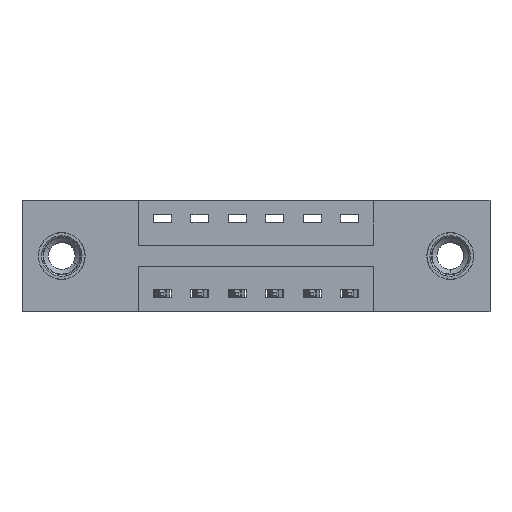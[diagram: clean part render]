
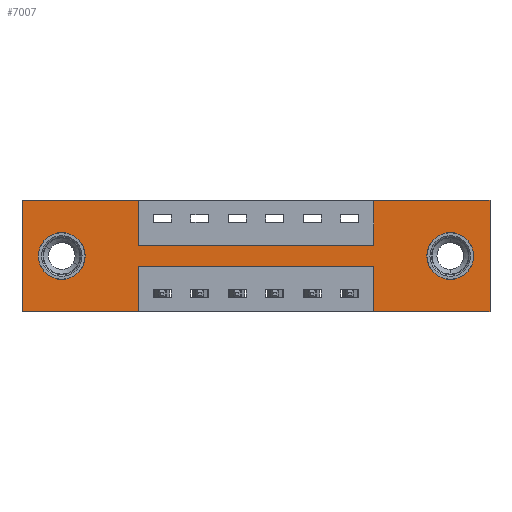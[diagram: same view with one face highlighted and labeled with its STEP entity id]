
A CAD part, front view. The second image highlights one B-rep face of the part: STEP entity #7007.
In plain terms, the highlighted planar face has unit normal (0, -1, 0).
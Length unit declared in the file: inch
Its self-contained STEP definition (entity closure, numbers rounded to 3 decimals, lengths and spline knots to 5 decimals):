
#60 = PLANE ( 'NONE',  #9162 ) ;
#218 = VERTEX_POINT ( 'NONE', #9192 ) ;
#221 = DIRECTION ( 'NONE',  ( 0., 0., 1. ) ) ;
#252 = AXIS2_PLACEMENT_3D ( 'NONE', #3395, #7339, #2103 ) ;
#494 = CARTESIAN_POINT ( 'NONE',  ( 1.56, 0., -0.37 ) ) ;
#575 = EDGE_CURVE ( 'NONE', #1447, #1108, #4317, .T. ) ;
#617 = DIRECTION ( 'NONE',  ( 0., 0., -1. ) ) ;
#659 = CARTESIAN_POINT ( 'NONE',  ( 0., 0., -0.37 ) ) ;
#671 = ORIENTED_EDGE ( 'NONE', *, *, #3765, .F. ) ;
#778 = ORIENTED_EDGE ( 'NONE', *, *, #8247, .F. ) ;
#977 = LINE ( 'NONE', #2435, #4681 ) ;
#992 = LINE ( 'NONE', #3208, #8016 ) ;
#1108 = VERTEX_POINT ( 'NONE', #1292 ) ;
#1255 = ORIENTED_EDGE ( 'NONE', *, *, #1481, .F. ) ;
#1270 = VECTOR ( 'NONE', #5062, 39.37008 ) ;
#1292 = CARTESIAN_POINT ( 'NONE',  ( 0.3875, 0., -0.37 ) ) ;
#1352 = VERTEX_POINT ( 'NONE', #8422 ) ;
#1397 = DIRECTION ( 'NONE',  ( -1., 0., 0. ) ) ;
#1408 = CARTESIAN_POINT ( 'NONE',  ( 1.4275, 0., -0.185 ) ) ;
#1447 = VERTEX_POINT ( 'NONE', #5711 ) ;
#1481 = EDGE_CURVE ( 'NONE', #1352, #1447, #5524, .T. ) ;
#1597 = CARTESIAN_POINT ( 'NONE',  ( 0.1325, 0., -0.107 ) ) ;
#1682 = CARTESIAN_POINT ( 'NONE',  ( 1.56, 0., 0. ) ) ;
#1745 = CIRCLE ( 'NONE', #7220, 0.078 ) ;
#1854 = CARTESIAN_POINT ( 'NONE',  ( 1.1725, 0., -0.37 ) ) ;
#1935 = CARTESIAN_POINT ( 'NONE',  ( 0.3875, 0., -0.15 ) ) ;
#1977 = DIRECTION ( 'NONE',  ( 0., 0., -1. ) ) ;
#2103 = DIRECTION ( 'NONE',  ( 0., 0., 1. ) ) ;
#2219 = VECTOR ( 'NONE', #9216, 39.37008 ) ;
#2435 = CARTESIAN_POINT ( 'NONE',  ( 1.1725, 0., 0. ) ) ;
#2485 = LINE ( 'NONE', #7800, #6066 ) ;
#2497 = DIRECTION ( 'NONE',  ( 0., 0., -1. ) ) ;
#2547 = VERTEX_POINT ( 'NONE', #1935 ) ;
#2572 = CARTESIAN_POINT ( 'NONE',  ( 0., 0., 0. ) ) ;
#2599 = ORIENTED_EDGE ( 'NONE', *, *, #575, .F. ) ;
#2664 = CARTESIAN_POINT ( 'NONE',  ( 0.1325, 0., -0.185 ) ) ;
#2705 = VECTOR ( 'NONE', #4104, 39.37008 ) ;
#2796 = VERTEX_POINT ( 'NONE', #7964 ) ;
#2830 = CIRCLE ( 'NONE', #8495, 0.078 ) ;
#2848 = AXIS2_PLACEMENT_3D ( 'NONE', #2664, #2879, #8687 ) ;
#2854 = CIRCLE ( 'NONE', #2848, 0.078 ) ;
#2879 = DIRECTION ( 'NONE',  ( 0., 1., 0. ) ) ;
#2963 = DIRECTION ( 'NONE',  ( 1., 0., 0. ) ) ;
#3015 = DIRECTION ( 'NONE',  ( 0., 0., -1. ) ) ;
#3023 = FACE_BOUND ( 'NONE', #6257, .T. ) ;
#3056 = DIRECTION ( 'NONE',  ( 0., -1., 0. ) ) ;
#3208 = CARTESIAN_POINT ( 'NONE',  ( 1.56, 0., 0. ) ) ;
#3235 = LINE ( 'NONE', #6125, #5086 ) ;
#3273 = EDGE_CURVE ( 'NONE', #9196, #5126, #992, .T. ) ;
#3340 = ORIENTED_EDGE ( 'NONE', *, *, #8353, .T. ) ;
#3395 = CARTESIAN_POINT ( 'NONE',  ( 0.1325, 0., -0.185 ) ) ;
#3583 = DIRECTION ( 'NONE',  ( 0., 1., 0. ) ) ;
#3716 = DIRECTION ( 'NONE',  ( 0., 1., 0. ) ) ;
#3764 = VECTOR ( 'NONE', #4928, 39.37008 ) ;
#3765 = EDGE_CURVE ( 'NONE', #7352, #6987, #977, .T. ) ;
#3979 = ORIENTED_EDGE ( 'NONE', *, *, #8558, .F. ) ;
#4104 = DIRECTION ( 'NONE',  ( 1., 0., 0. ) ) ;
#4143 = EDGE_CURVE ( 'NONE', #218, #4602, #1745, .T. ) ;
#4197 = ORIENTED_EDGE ( 'NONE', *, *, #7947, .F. ) ;
#4316 = VERTEX_POINT ( 'NONE', #9647 ) ;
#4317 = LINE ( 'NONE', #9525, #4801 ) ;
#4602 = VERTEX_POINT ( 'NONE', #5393 ) ;
#4681 = VECTOR ( 'NONE', #5429, 39.37008 ) ;
#4735 = ORIENTED_EDGE ( 'NONE', *, *, #5705, .F. ) ;
#4768 = VERTEX_POINT ( 'NONE', #1854 ) ;
#4800 = DIRECTION ( 'NONE',  ( -1., 0., 0. ) ) ;
#4801 = VECTOR ( 'NONE', #1977, 39.37008 ) ;
#4901 = EDGE_CURVE ( 'NONE', #5126, #4768, #8763, .T. ) ;
#4928 = DIRECTION ( 'NONE',  ( 0., 0., 1. ) ) ;
#5058 = DIRECTION ( 'NONE',  ( 0., 0., -1. ) ) ;
#5062 = DIRECTION ( 'NONE',  ( -1., 0., 0. ) ) ;
#5070 = ORIENTED_EDGE ( 'NONE', *, *, #6758, .F. ) ;
#5086 = VECTOR ( 'NONE', #4800, 39.37008 ) ;
#5126 = VERTEX_POINT ( 'NONE', #494 ) ;
#5177 = CARTESIAN_POINT ( 'NONE',  ( 0., 0., -0.37 ) ) ;
#5393 = CARTESIAN_POINT ( 'NONE',  ( 1.4275, 0., -0.263 ) ) ;
#5397 = LINE ( 'NONE', #2572, #2705 ) ;
#5429 = DIRECTION ( 'NONE',  ( 0., 0., 1. ) ) ;
#5437 = CARTESIAN_POINT ( 'NONE',  ( 0., 0., 0. ) ) ;
#5524 = LINE ( 'NONE', #8703, #1270 ) ;
#5705 = EDGE_CURVE ( 'NONE', #4768, #1352, #2485, .T. ) ;
#5711 = CARTESIAN_POINT ( 'NONE',  ( 0.3875, 0., -0.22 ) ) ;
#5747 = LINE ( 'NONE', #7272, #6718 ) ;
#5859 = CARTESIAN_POINT ( 'NONE',  ( 0., 0., 0. ) ) ;
#5994 = CARTESIAN_POINT ( 'NONE',  ( 0., 0., -0.37 ) ) ;
#6066 = VECTOR ( 'NONE', #221, 39.37008 ) ;
#6119 = ORIENTED_EDGE ( 'NONE', *, *, #8307, .T. ) ;
#6123 = CARTESIAN_POINT ( 'NONE',  ( 0.3875, 0., -0.15 ) ) ;
#6125 = CARTESIAN_POINT ( 'NONE',  ( 0., 0., -0.37 ) ) ;
#6252 = VERTEX_POINT ( 'NONE', #5177 ) ;
#6257 = EDGE_LOOP ( 'NONE', ( #8660, #6119 ) ) ;
#6309 = VERTEX_POINT ( 'NONE', #1597 ) ;
#6491 = CIRCLE ( 'NONE', #252, 0.078 ) ;
#6632 = FACE_BOUND ( 'NONE', #8911, .T. ) ;
#6718 = VECTOR ( 'NONE', #5058, 39.37008 ) ;
#6758 = EDGE_CURVE ( 'NONE', #2796, #7705, #5397, .T. ) ;
#6793 = CARTESIAN_POINT ( 'NONE',  ( 0.3875, 0., 0. ) ) ;
#6908 = VECTOR ( 'NONE', #1397, 39.37008 ) ;
#6987 = VERTEX_POINT ( 'NONE', #9677 ) ;
#7007 = ADVANCED_FACE ( 'NONE', ( #3023, #6632, #8223 ), #60, .T. ) ;
#7141 = ORIENTED_EDGE ( 'NONE', *, *, #9787, .F. ) ;
#7210 = EDGE_LOOP ( 'NONE', ( #2599, #1255, #4735, #9708, #9101, #778, #671, #7141, #4197, #5070, #8939, #3979 ) ) ;
#7220 = AXIS2_PLACEMENT_3D ( 'NONE', #1408, #3716, #3015 ) ;
#7272 = CARTESIAN_POINT ( 'NONE',  ( 0.3875, 0., 0. ) ) ;
#7339 = DIRECTION ( 'NONE',  ( 0., 1., 0. ) ) ;
#7352 = VERTEX_POINT ( 'NONE', #7625 ) ;
#7364 = LINE ( 'NONE', #5859, #3764 ) ;
#7625 = CARTESIAN_POINT ( 'NONE',  ( 1.1725, 0., -0.15 ) ) ;
#7634 = LINE ( 'NONE', #6123, #7896 ) ;
#7641 = EDGE_CURVE ( 'NONE', #6252, #2796, #7364, .T. ) ;
#7705 = VERTEX_POINT ( 'NONE', #6793 ) ;
#7800 = CARTESIAN_POINT ( 'NONE',  ( 1.1725, 0., -0.37 ) ) ;
#7896 = VECTOR ( 'NONE', #2963, 39.37008 ) ;
#7947 = EDGE_CURVE ( 'NONE', #7705, #2547, #5747, .T. ) ;
#7964 = CARTESIAN_POINT ( 'NONE',  ( 0., 0., 0. ) ) ;
#8016 = VECTOR ( 'NONE', #2497, 39.37008 ) ;
#8165 = DIRECTION ( 'NONE',  ( 0., 0., -1. ) ) ;
#8223 = FACE_OUTER_BOUND ( 'NONE', #7210, .T. ) ;
#8247 = EDGE_CURVE ( 'NONE', #6987, #9196, #9422, .T. ) ;
#8307 = EDGE_CURVE ( 'NONE', #4602, #218, #2830, .T. ) ;
#8353 = EDGE_CURVE ( 'NONE', #4316, #6309, #6491, .T. ) ;
#8422 = CARTESIAN_POINT ( 'NONE',  ( 1.1725, 0., -0.22 ) ) ;
#8495 = AXIS2_PLACEMENT_3D ( 'NONE', #8821, #3583, #617 ) ;
#8558 = EDGE_CURVE ( 'NONE', #1108, #6252, #3235, .T. ) ;
#8660 = ORIENTED_EDGE ( 'NONE', *, *, #4143, .T. ) ;
#8687 = DIRECTION ( 'NONE',  ( 0., 0., 1. ) ) ;
#8703 = CARTESIAN_POINT ( 'NONE',  ( 0.3875, 0., -0.22 ) ) ;
#8763 = LINE ( 'NONE', #659, #6908 ) ;
#8821 = CARTESIAN_POINT ( 'NONE',  ( 1.4275, 0., -0.185 ) ) ;
#8856 = ORIENTED_EDGE ( 'NONE', *, *, #9645, .T. ) ;
#8911 = EDGE_LOOP ( 'NONE', ( #8856, #3340 ) ) ;
#8939 = ORIENTED_EDGE ( 'NONE', *, *, #7641, .F. ) ;
#9101 = ORIENTED_EDGE ( 'NONE', *, *, #3273, .F. ) ;
#9162 = AXIS2_PLACEMENT_3D ( 'NONE', #5994, #3056, #8165 ) ;
#9192 = CARTESIAN_POINT ( 'NONE',  ( 1.4275, 0., -0.107 ) ) ;
#9196 = VERTEX_POINT ( 'NONE', #1682 ) ;
#9216 = DIRECTION ( 'NONE',  ( 1., 0., 0. ) ) ;
#9422 = LINE ( 'NONE', #5437, #2219 ) ;
#9525 = CARTESIAN_POINT ( 'NONE',  ( 0.3875, 0., -0.37 ) ) ;
#9645 = EDGE_CURVE ( 'NONE', #6309, #4316, #2854, .T. ) ;
#9647 = CARTESIAN_POINT ( 'NONE',  ( 0.1325, 0., -0.263 ) ) ;
#9677 = CARTESIAN_POINT ( 'NONE',  ( 1.1725, 0., 0. ) ) ;
#9708 = ORIENTED_EDGE ( 'NONE', *, *, #4901, .F. ) ;
#9787 = EDGE_CURVE ( 'NONE', #2547, #7352, #7634, .T. ) ;
